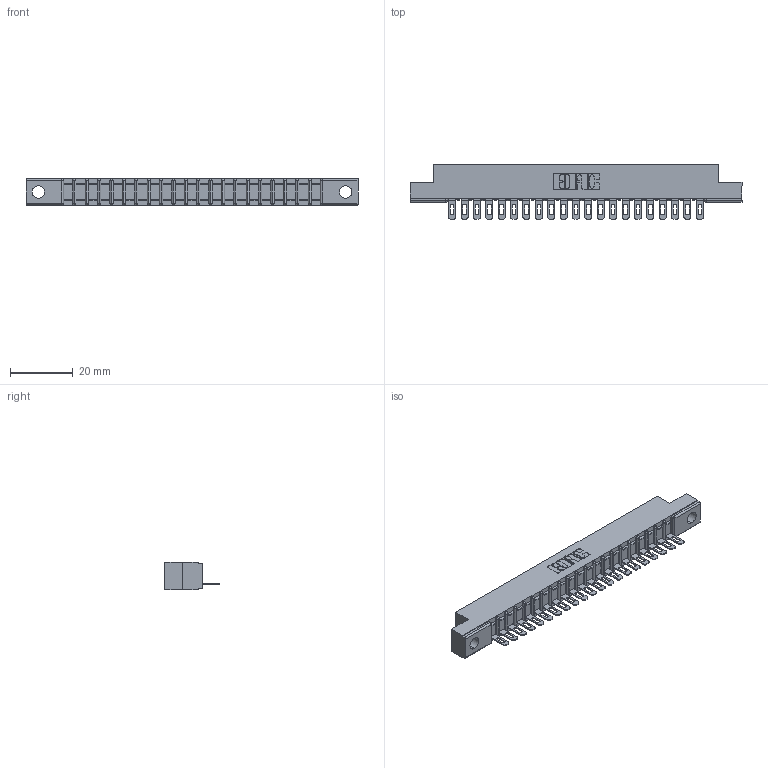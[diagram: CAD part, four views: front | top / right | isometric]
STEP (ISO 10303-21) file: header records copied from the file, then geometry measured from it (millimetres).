
FILE_DESCRIPTION (( 'STEP AP203' ), '1' );
FILE_NAME ('307-021-501-102.STEP', '2019-09-04T23:23:14', ( '' ), ( '' ), 'SwSTEP 2.0', 'SolidWorks 2016', '' );
FILE_SCHEMA (( 'CONFIG_CONTROL_DESIGN' ));
Length unit declared in the file: inch
Products named in the file (3): 307 Part_.128 Dia Mounting Holes; 307-021-501-102; 307-290-002_501
Assembly tree (22 placements, depth 2):
  307-021-501-102
    307 Part_.128 Dia Mounting Holes
    307-290-002_501  x21
Bounding box: 106.22 x 17.42 x 8.71 mm (x, y, z)
Volume: 6942.5 mm3; surface area: 12561.2 mm2
Topology: 22 solids, 22 shells, 1736 faces, 5321 edges, 3486 vertices
Faces by surface type: plane 994, cylinder 698, sphere 44
Entity records: 21388 total; most frequent: CARTESIAN_POINT 3604, ORIENTED_EDGE 3594, DIRECTION 3515, EDGE_CURVE 1797, VECTOR 1361, LINE 1361, VERTEX_POINT 1166, AXIS2_PLACEMENT_3D 1077
